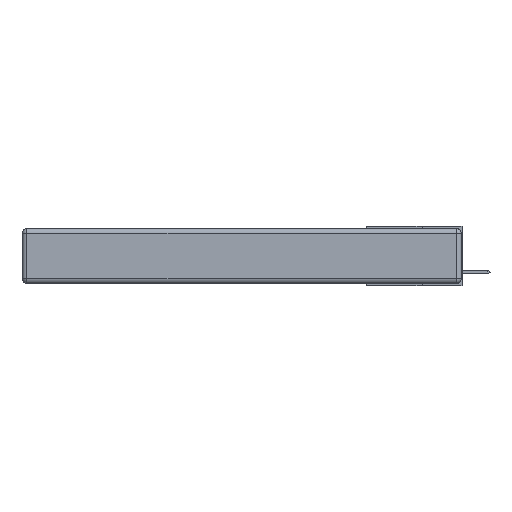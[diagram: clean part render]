
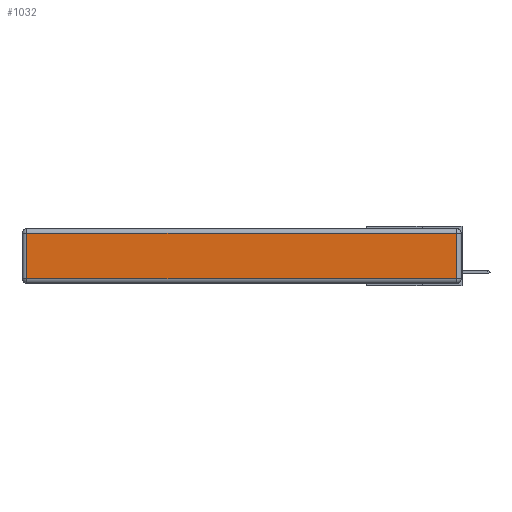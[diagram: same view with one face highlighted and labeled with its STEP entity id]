
A CAD part, left-side view. The second image highlights one B-rep face of the part: STEP entity #1032.
In plain terms, the highlighted planar face has unit normal (-1, 0, 0).
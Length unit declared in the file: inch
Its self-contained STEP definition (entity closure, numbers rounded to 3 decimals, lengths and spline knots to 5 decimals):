
#160 = EDGE_CURVE ( 'NONE', #26552, #3177, #10286, .T. ) ;
#1032 = ADVANCED_FACE ( 'NONE', ( #3325 ), #12032, .T. ) ;
#2937 = DIRECTION ( 'NONE',  ( 0., 0., -1. ) ) ;
#3031 = CARTESIAN_POINT ( 'NONE',  ( 0., 0., -0.313 ) ) ;
#3111 = CARTESIAN_POINT ( 'NONE',  ( 0., 0.03, -0.313 ) ) ;
#3177 = VERTEX_POINT ( 'NONE', #3111 ) ;
#3325 = FACE_OUTER_BOUND ( 'NONE', #20449, .T. ) ;
#3423 = VECTOR ( 'NONE', #18444, 39.37008 ) ;
#3871 = DIRECTION ( 'NONE',  ( 0., 1., 0. ) ) ;
#6723 = VECTOR ( 'NONE', #23879, 39.37008 ) ;
#6900 = VECTOR ( 'NONE', #3871, 39.37008 ) ;
#7259 = EDGE_CURVE ( 'NONE', #29380, #26552, #16715, .T. ) ;
#10286 = LINE ( 'NONE', #3031, #3423 ) ;
#10855 = CARTESIAN_POINT ( 'NONE',  ( 0., 2.72, -0.343 ) ) ;
#12032 = PLANE ( 'NONE',  #30446 ) ;
#16715 = LINE ( 'NONE', #10855, #27222 ) ;
#17192 = ORIENTED_EDGE ( 'NONE', *, *, #31892, .T. ) ;
#17453 = ORIENTED_EDGE ( 'NONE', *, *, #160, .T. ) ;
#17527 = CARTESIAN_POINT ( 'NONE',  ( 0., 2.72, -0.03 ) ) ;
#18444 = DIRECTION ( 'NONE',  ( 0., -1., 0. ) ) ;
#19045 = LINE ( 'NONE', #32185, #6900 ) ;
#20449 = EDGE_LOOP ( 'NONE', ( #17453, #17192, #31277, #21338 ) ) ;
#21338 = ORIENTED_EDGE ( 'NONE', *, *, #7259, .T. ) ;
#22854 = CARTESIAN_POINT ( 'NONE',  ( 0., 0.03, -0.03 ) ) ;
#23879 = DIRECTION ( 'NONE',  ( 0., 0., 1. ) ) ;
#24592 = DIRECTION ( 'NONE',  ( 0., 0., 1. ) ) ;
#25048 = DIRECTION ( 'NONE',  ( -1., 0., 0. ) ) ;
#26552 = VERTEX_POINT ( 'NONE', #27357 ) ;
#27222 = VECTOR ( 'NONE', #2937, 39.37008 ) ;
#27357 = CARTESIAN_POINT ( 'NONE',  ( 0., 2.72, -0.313 ) ) ;
#28147 = LINE ( 'NONE', #31191, #6723 ) ;
#28782 = EDGE_CURVE ( 'NONE', #31641, #29380, #19045, .T. ) ;
#29380 = VERTEX_POINT ( 'NONE', #17527 ) ;
#30446 = AXIS2_PLACEMENT_3D ( 'NONE', #32646, #25048, #24592 ) ;
#31191 = CARTESIAN_POINT ( 'NONE',  ( 0., 0.03, -0.343 ) ) ;
#31277 = ORIENTED_EDGE ( 'NONE', *, *, #28782, .T. ) ;
#31641 = VERTEX_POINT ( 'NONE', #22854 ) ;
#31892 = EDGE_CURVE ( 'NONE', #3177, #31641, #28147, .T. ) ;
#32185 = CARTESIAN_POINT ( 'NONE',  ( 0., 2.75, -0.03 ) ) ;
#32646 = CARTESIAN_POINT ( 'NONE',  ( 0., 0., -0.343 ) ) ;
